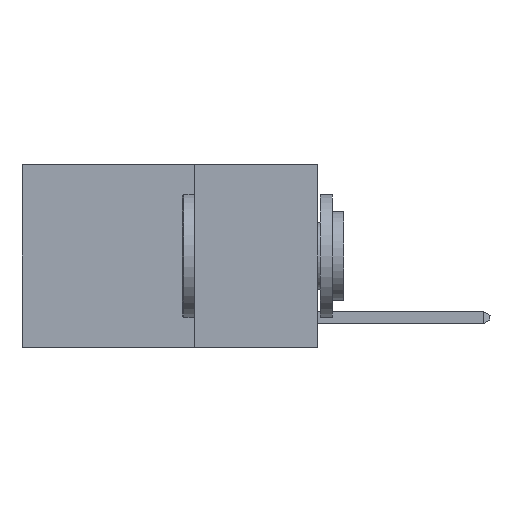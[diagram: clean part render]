
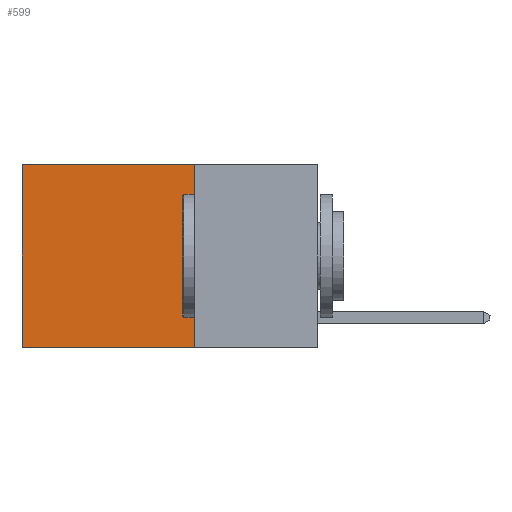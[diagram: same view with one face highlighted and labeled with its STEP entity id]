
A CAD part, left-side view. The second image highlights one B-rep face of the part: STEP entity #599.
In plain terms, the highlighted planar face has unit normal (-1, 0, 0).
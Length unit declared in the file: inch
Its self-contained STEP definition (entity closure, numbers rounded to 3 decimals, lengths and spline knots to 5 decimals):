
#429 = EDGE_CURVE ( 'NONE', #20386, #17868, #29378, .T. ) ;
#599 = ADVANCED_FACE ( 'NONE', ( #28661 ), #26684, .F. ) ;
#653 = CARTESIAN_POINT ( 'NONE',  ( 0.2625, 0.25, 0. ) ) ;
#1204 = VECTOR ( 'NONE', #17973, 39.37008 ) ;
#2286 = VECTOR ( 'NONE', #27414, 39.37008 ) ;
#7128 = ORIENTED_EDGE ( 'NONE', *, *, #24327, .F. ) ;
#8039 = LINE ( 'NONE', #13456, #2286 ) ;
#9114 = ORIENTED_EDGE ( 'NONE', *, *, #429, .T. ) ;
#9689 = VECTOR ( 'NONE', #18776, 39.37008 ) ;
#10429 = EDGE_CURVE ( 'NONE', #26201, #17868, #8039, .T. ) ;
#10638 = CARTESIAN_POINT ( 'NONE',  ( 0.2625, 0.25, 0. ) ) ;
#11010 = LINE ( 'NONE', #653, #23954 ) ;
#11061 = CARTESIAN_POINT ( 'NONE',  ( 0.2625, 0.25, 0. ) ) ;
#13364 = ORIENTED_EDGE ( 'NONE', *, *, #10429, .F. ) ;
#13456 = CARTESIAN_POINT ( 'NONE',  ( 0.2625, 0.25, -0.37 ) ) ;
#14285 = EDGE_LOOP ( 'NONE', ( #9114, #13364, #7128, #19184 ) ) ;
#16302 = VERTEX_POINT ( 'NONE', #29667 ) ;
#16642 = CARTESIAN_POINT ( 'NONE',  ( 0.2625, 0.6, 0. ) ) ;
#17868 = VERTEX_POINT ( 'NONE', #18121 ) ;
#17973 = DIRECTION ( 'NONE',  ( 0., 1., 0. ) ) ;
#18121 = CARTESIAN_POINT ( 'NONE',  ( 0.2625, 0.6, -0.37 ) ) ;
#18776 = DIRECTION ( 'NONE',  ( 0., 0., -1. ) ) ;
#18889 = AXIS2_PLACEMENT_3D ( 'NONE', #10638, #22290, #28857 ) ;
#19184 = ORIENTED_EDGE ( 'NONE', *, *, #20366, .T. ) ;
#20366 = EDGE_CURVE ( 'NONE', #16302, #20386, #22416, .T. ) ;
#20386 = VERTEX_POINT ( 'NONE', #27777 ) ;
#21317 = DIRECTION ( 'NONE',  ( 0., 0., -1. ) ) ;
#22290 = DIRECTION ( 'NONE',  ( 1., 0., 0. ) ) ;
#22416 = LINE ( 'NONE', #11061, #1204 ) ;
#22432 = CARTESIAN_POINT ( 'NONE',  ( 0.2625, 0.25, -0.37 ) ) ;
#23954 = VECTOR ( 'NONE', #21317, 39.37008 ) ;
#24327 = EDGE_CURVE ( 'NONE', #16302, #26201, #11010, .T. ) ;
#26201 = VERTEX_POINT ( 'NONE', #22432 ) ;
#26684 = PLANE ( 'NONE',  #18889 ) ;
#27414 = DIRECTION ( 'NONE',  ( 0., 1., 0. ) ) ;
#27777 = CARTESIAN_POINT ( 'NONE',  ( 0.2625, 0.6, 0. ) ) ;
#28661 = FACE_OUTER_BOUND ( 'NONE', #14285, .T. ) ;
#28857 = DIRECTION ( 'NONE',  ( 0., 0., -1. ) ) ;
#29378 = LINE ( 'NONE', #16642, #9689 ) ;
#29667 = CARTESIAN_POINT ( 'NONE',  ( 0.2625, 0.25, 0. ) ) ;
